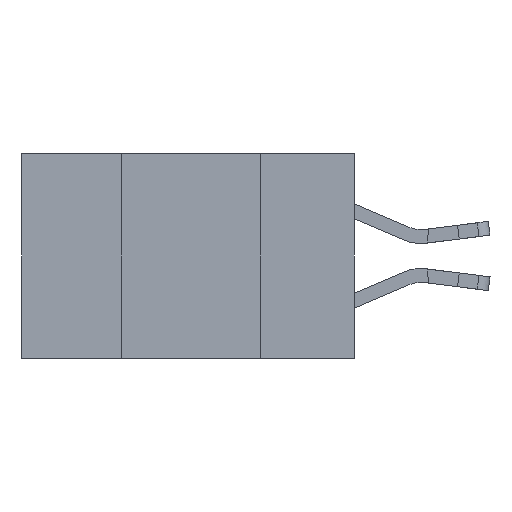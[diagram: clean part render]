
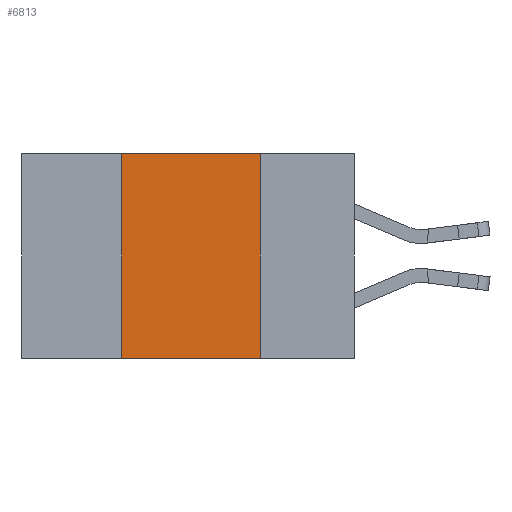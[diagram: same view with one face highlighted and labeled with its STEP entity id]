
A CAD part, left-side view. The second image highlights one B-rep face of the part: STEP entity #6813.
In plain terms, the highlighted planar face has unit normal (-1, 0, 0).
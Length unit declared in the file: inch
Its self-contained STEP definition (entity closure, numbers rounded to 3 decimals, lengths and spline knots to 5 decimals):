
#77 = CARTESIAN_POINT ( 'NONE',  ( 0., 0.42, -0.37 ) ) ;
#112 = LINE ( 'NONE', #10235, #16034 ) ;
#206 = EDGE_CURVE ( 'NONE', #7160, #12007, #17663, .T. ) ;
#930 = DIRECTION ( 'NONE',  ( 0., 0., -1. ) ) ;
#1434 = CARTESIAN_POINT ( 'NONE',  ( 0., 0.17, 0. ) ) ;
#1601 = EDGE_CURVE ( 'NONE', #13930, #5735, #112, .T. ) ;
#2306 = FACE_OUTER_BOUND ( 'NONE', #4529, .T. ) ;
#2545 = VECTOR ( 'NONE', #15773, 39.37008 ) ;
#2925 = EDGE_CURVE ( 'NONE', #12007, #5735, #15066, .T. ) ;
#2998 = EDGE_CURVE ( 'NONE', #13930, #7160, #3919, .T. ) ;
#3919 = LINE ( 'NONE', #10273, #2545 ) ;
#4492 = ORIENTED_EDGE ( 'NONE', *, *, #2998, .F. ) ;
#4529 = EDGE_LOOP ( 'NONE', ( #14297, #9514, #4492, #8690 ) ) ;
#5588 = VECTOR ( 'NONE', #17151, 39.37008 ) ;
#5735 = VERTEX_POINT ( 'NONE', #15453 ) ;
#6813 = ADVANCED_FACE ( 'NONE', ( #2306 ), #9725, .F. ) ;
#7160 = VERTEX_POINT ( 'NONE', #17694 ) ;
#8306 = DIRECTION ( 'NONE',  ( 1., 0., 0. ) ) ;
#8690 = ORIENTED_EDGE ( 'NONE', *, *, #1601, .T. ) ;
#9514 = ORIENTED_EDGE ( 'NONE', *, *, #206, .F. ) ;
#9725 = PLANE ( 'NONE',  #12079 ) ;
#10235 = CARTESIAN_POINT ( 'NONE',  ( 0., 0.6, -0.37 ) ) ;
#10273 = CARTESIAN_POINT ( 'NONE',  ( 0., 0.42, 0. ) ) ;
#10409 = DIRECTION ( 'NONE',  ( 0., 0., -1. ) ) ;
#11213 = VECTOR ( 'NONE', #10409, 39.37008 ) ;
#12007 = VERTEX_POINT ( 'NONE', #18767 ) ;
#12079 = AXIS2_PLACEMENT_3D ( 'NONE', #17026, #8306, #930 ) ;
#13930 = VERTEX_POINT ( 'NONE', #77 ) ;
#14297 = ORIENTED_EDGE ( 'NONE', *, *, #2925, .F. ) ;
#14690 = CARTESIAN_POINT ( 'NONE',  ( 0., 0.6, 0. ) ) ;
#15066 = LINE ( 'NONE', #1434, #11213 ) ;
#15453 = CARTESIAN_POINT ( 'NONE',  ( 0., 0.17, -0.37 ) ) ;
#15773 = DIRECTION ( 'NONE',  ( 0., 0., 1. ) ) ;
#16034 = VECTOR ( 'NONE', #17460, 39.37008 ) ;
#17026 = CARTESIAN_POINT ( 'NONE',  ( 0., 0.6, 0. ) ) ;
#17151 = DIRECTION ( 'NONE',  ( 0., -1., 0. ) ) ;
#17460 = DIRECTION ( 'NONE',  ( 0., -1., 0. ) ) ;
#17663 = LINE ( 'NONE', #14690, #5588 ) ;
#17694 = CARTESIAN_POINT ( 'NONE',  ( 0., 0.42, 0. ) ) ;
#18767 = CARTESIAN_POINT ( 'NONE',  ( 0., 0.17, 0. ) ) ;
